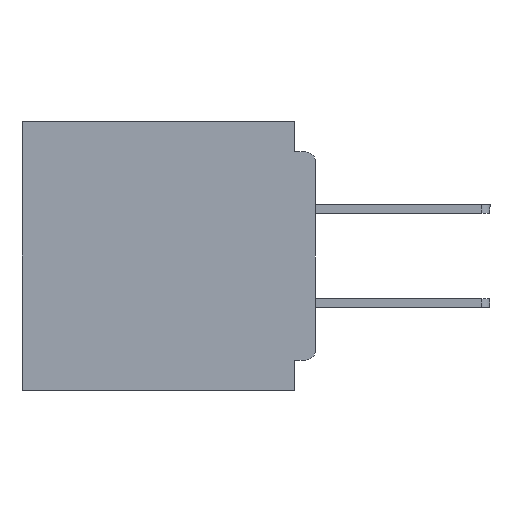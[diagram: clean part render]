
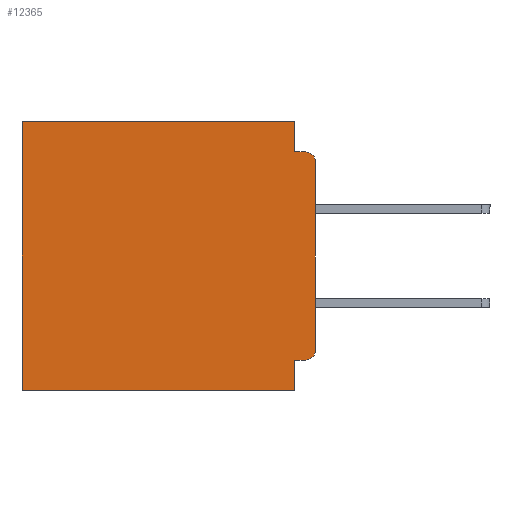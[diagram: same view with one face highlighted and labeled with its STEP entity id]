
A CAD part, left-side view. The second image highlights one B-rep face of the part: STEP entity #12365.
In plain terms, the highlighted planar face has unit normal (-1, 0, 0).
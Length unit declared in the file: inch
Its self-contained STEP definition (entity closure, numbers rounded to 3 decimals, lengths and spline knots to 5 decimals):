
#610 = ORIENTED_EDGE ( 'NONE', *, *, #2896, .F. ) ;
#1330 = CARTESIAN_POINT ( 'NONE',  ( 0.3, 0., -0.4 ) ) ;
#1435 = DIRECTION ( 'NONE',  ( 0., 1., 0. ) ) ;
#1520 = ORIENTED_EDGE ( 'NONE', *, *, #22084, .F. ) ;
#1573 = DIRECTION ( 'NONE',  ( 0., 0., -1. ) ) ;
#1680 = VECTOR ( 'NONE', #18520, 39.37008 ) ;
#2896 = EDGE_CURVE ( 'NONE', #43813, #3891, #23400, .T. ) ;
#2924 = CARTESIAN_POINT ( 'NONE',  ( 0.3, 0., -0.06 ) ) ;
#3100 = EDGE_CURVE ( 'NONE', #37836, #30826, #6459, .T. ) ;
#3891 = VERTEX_POINT ( 'NONE', #12696 ) ;
#4060 = DIRECTION ( 'NONE',  ( 0., 0., -1. ) ) ;
#4715 = LINE ( 'NONE', #31623, #22183 ) ;
#5280 = LINE ( 'NONE', #23691, #22742 ) ;
#5932 = VERTEX_POINT ( 'NONE', #44274 ) ;
#6318 = DIRECTION ( 'NONE',  ( 0., 1., 0. ) ) ;
#6379 = FACE_OUTER_BOUND ( 'NONE', #38241, .T. ) ;
#6459 = LINE ( 'NONE', #1330, #14608 ) ;
#7271 = DIRECTION ( 'NONE',  ( 0., 1., 0. ) ) ;
#8117 = EDGE_CURVE ( 'NONE', #28402, #30826, #22431, .T. ) ;
#8586 = ORIENTED_EDGE ( 'NONE', *, *, #20855, .T. ) ;
#9875 = VERTEX_POINT ( 'NONE', #26850 ) ;
#11197 = DIRECTION ( 'NONE',  ( 0., 0., -1. ) ) ;
#11500 = CARTESIAN_POINT ( 'NONE',  ( 0.3, 0., -0.4 ) ) ;
#11609 = CARTESIAN_POINT ( 'NONE',  ( 0.3, 0.437, 0. ) ) ;
#12365 = ADVANCED_FACE ( 'NONE', ( #6379 ), #18963, .F. ) ;
#12696 = CARTESIAN_POINT ( 'NONE',  ( 0.3, 0., -0.34 ) ) ;
#13729 = CARTESIAN_POINT ( 'NONE',  ( 0.3, 0., -0.045 ) ) ;
#13941 = EDGE_CURVE ( 'NONE', #43813, #41129, #39469, .T. ) ;
#14608 = VECTOR ( 'NONE', #1435, 39.37008 ) ;
#14794 = ORIENTED_EDGE ( 'NONE', *, *, #24269, .T. ) ;
#16261 = VERTEX_POINT ( 'NONE', #19914 ) ;
#16430 = ORIENTED_EDGE ( 'NONE', *, *, #13941, .T. ) ;
#17509 = DIRECTION ( 'NONE',  ( -1., 0., 0. ) ) ;
#18220 = CARTESIAN_POINT ( 'NONE',  ( 0.3, 0.015, -0.06 ) ) ;
#18520 = DIRECTION ( 'NONE',  ( 0., 0., -1. ) ) ;
#18963 = PLANE ( 'NONE',  #21961 ) ;
#19072 = AXIS2_PLACEMENT_3D ( 'NONE', #18220, #42579, #21732 ) ;
#19914 = CARTESIAN_POINT ( 'NONE',  ( 0.3, 0.031, -0.045 ) ) ;
#20855 = EDGE_CURVE ( 'NONE', #5932, #3891, #41547, .T. ) ;
#21732 = DIRECTION ( 'NONE',  ( 0., 0., -1. ) ) ;
#21961 = AXIS2_PLACEMENT_3D ( 'NONE', #29145, #22482, #1573 ) ;
#22084 = EDGE_CURVE ( 'NONE', #16261, #41129, #44689, .T. ) ;
#22183 = VECTOR ( 'NONE', #7271, 39.37008 ) ;
#22431 = LINE ( 'NONE', #29003, #1680 ) ;
#22482 = DIRECTION ( 'NONE',  ( 1., 0., 0. ) ) ;
#22742 = VECTOR ( 'NONE', #6318, 39.37008 ) ;
#22782 = VECTOR ( 'NONE', #11197, 39.37008 ) ;
#23106 = AXIS2_PLACEMENT_3D ( 'NONE', #38359, #17509, #41870 ) ;
#23400 = LINE ( 'NONE', #11500, #31539 ) ;
#23691 = CARTESIAN_POINT ( 'NONE',  ( 0.3, 0., -0.355 ) ) ;
#23870 = VERTEX_POINT ( 'NONE', #25427 ) ;
#24269 = EDGE_CURVE ( 'NONE', #23870, #28402, #4715, .T. ) ;
#25093 = VECTOR ( 'NONE', #41614, 39.37008 ) ;
#25427 = CARTESIAN_POINT ( 'NONE',  ( 0.3, 0.031, 0. ) ) ;
#26850 = CARTESIAN_POINT ( 'NONE',  ( 0.3, 0.031, -0.355 ) ) ;
#27849 = ORIENTED_EDGE ( 'NONE', *, *, #37895, .F. ) ;
#28402 = VERTEX_POINT ( 'NONE', #11609 ) ;
#28990 = ORIENTED_EDGE ( 'NONE', *, *, #8117, .T. ) ;
#29003 = CARTESIAN_POINT ( 'NONE',  ( 0.3, 0.437, -0.4 ) ) ;
#29145 = CARTESIAN_POINT ( 'NONE',  ( 0.3, 0., -0.4 ) ) ;
#29776 = VECTOR ( 'NONE', #4060, 39.37008 ) ;
#30527 = ORIENTED_EDGE ( 'NONE', *, *, #33811, .F. ) ;
#30826 = VERTEX_POINT ( 'NONE', #33930 ) ;
#31494 = CARTESIAN_POINT ( 'NONE',  ( 0.3, 0.031, -0.4 ) ) ;
#31539 = VECTOR ( 'NONE', #39403, 39.37008 ) ;
#31623 = CARTESIAN_POINT ( 'NONE',  ( 0.3, 0., 0. ) ) ;
#33422 = EDGE_CURVE ( 'NONE', #23870, #16261, #42369, .T. ) ;
#33811 = EDGE_CURVE ( 'NONE', #5932, #9875, #5280, .T. ) ;
#33930 = CARTESIAN_POINT ( 'NONE',  ( 0.3, 0.437, -0.4 ) ) ;
#37069 = ORIENTED_EDGE ( 'NONE', *, *, #3100, .F. ) ;
#37836 = VERTEX_POINT ( 'NONE', #31494 ) ;
#37895 = EDGE_CURVE ( 'NONE', #9875, #37836, #39037, .T. ) ;
#38241 = EDGE_LOOP ( 'NONE', ( #610, #16430, #1520, #43052, #14794, #28990, #37069, #27849, #30527, #8586 ) ) ;
#38359 = CARTESIAN_POINT ( 'NONE',  ( 0.3, 0.015, -0.34 ) ) ;
#38806 = CARTESIAN_POINT ( 'NONE',  ( 0.3, 0.031, -0.4 ) ) ;
#39037 = LINE ( 'NONE', #38806, #29776 ) ;
#39403 = DIRECTION ( 'NONE',  ( 0., 0., -1. ) ) ;
#39428 = CARTESIAN_POINT ( 'NONE',  ( 0.3, 0.015, -0.045 ) ) ;
#39469 = CIRCLE ( 'NONE', #19072, 0.015 ) ;
#41129 = VERTEX_POINT ( 'NONE', #39428 ) ;
#41547 = CIRCLE ( 'NONE', #23106, 0.015 ) ;
#41614 = DIRECTION ( 'NONE',  ( 0., -1., 0. ) ) ;
#41870 = DIRECTION ( 'NONE',  ( 0., 0., -1. ) ) ;
#42369 = LINE ( 'NONE', #42439, #22782 ) ;
#42439 = CARTESIAN_POINT ( 'NONE',  ( 0.3, 0.031, 0. ) ) ;
#42579 = DIRECTION ( 'NONE',  ( -1., 0., 0. ) ) ;
#43052 = ORIENTED_EDGE ( 'NONE', *, *, #33422, .F. ) ;
#43813 = VERTEX_POINT ( 'NONE', #2924 ) ;
#44274 = CARTESIAN_POINT ( 'NONE',  ( 0.3, 0.015, -0.355 ) ) ;
#44689 = LINE ( 'NONE', #13729, #25093 ) ;
